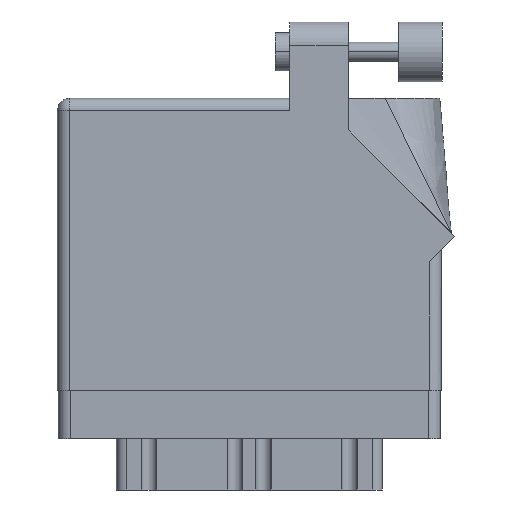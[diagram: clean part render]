
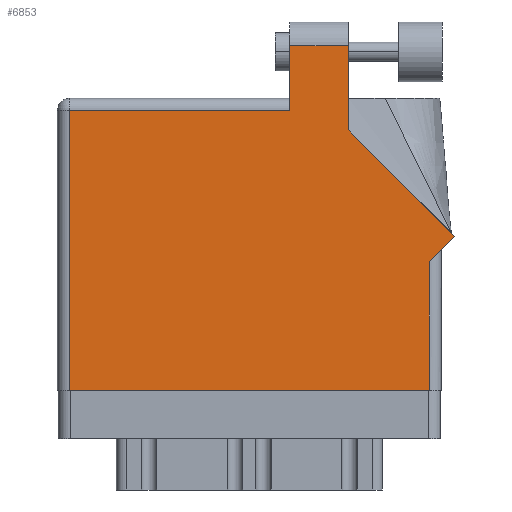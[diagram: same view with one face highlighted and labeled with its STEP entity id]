
A CAD part, front view. The second image highlights one B-rep face of the part: STEP entity #6853.
In plain terms, the highlighted face is planar.
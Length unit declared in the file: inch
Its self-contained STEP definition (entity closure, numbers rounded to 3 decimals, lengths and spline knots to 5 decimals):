
#353 = CARTESIAN_POINT ( 'NONE',  ( 1.948, 0.737, 0. ) ) ;
#829 = EDGE_CURVE ( 'NONE', #38516, #25380, #16410, .T. ) ;
#2902 = DIRECTION ( 'NONE',  ( 0., 1., 0. ) ) ;
#3990 = LINE ( 'NONE', #10843, #8149 ) ;
#4047 = DIRECTION ( 'NONE',  ( 0., -1., 0. ) ) ;
#4136 = EDGE_CURVE ( 'NONE', #24967, #4678, #3990, .T. ) ;
#4527 = VECTOR ( 'NONE', #28028, 39.37008 ) ;
#4678 = VERTEX_POINT ( 'NONE', #18419 ) ;
#5906 = EDGE_CURVE ( 'NONE', #9561, #29382, #34043, .T. ) ;
#6853 = ADVANCED_FACE ( 'NONE', ( #13841 ), #32233, .F. ) ;
#6897 = AXIS2_PLACEMENT_3D ( 'NONE', #11452, #38117, #23418 ) ;
#7195 = CARTESIAN_POINT ( 'NONE',  ( 2.01, 0.737, 0. ) ) ;
#7504 = ORIENTED_EDGE ( 'NONE', *, *, #23380, .T. ) ;
#7638 = LINE ( 'NONE', #16473, #4527 ) ;
#7779 = DIRECTION ( 'NONE',  ( 0., 1., 0. ) ) ;
#8149 = VECTOR ( 'NONE', #25350, 39.37008 ) ;
#8439 = CARTESIAN_POINT ( 'NONE',  ( 1.217, 1.805, 0. ) ) ;
#8461 = ORIENTED_EDGE ( 'NONE', *, *, #4136, .T. ) ;
#9418 = VECTOR ( 'NONE', #7779, 39.37008 ) ;
#9561 = VERTEX_POINT ( 'NONE', #8439 ) ;
#9796 = VECTOR ( 'NONE', #33236, 39.37008 ) ;
#10843 = CARTESIAN_POINT ( 'NONE',  ( 0.062, 0., 0. ) ) ;
#11318 = CARTESIAN_POINT ( 'NONE',  ( 1.948, 0.675, 0. ) ) ;
#11452 = CARTESIAN_POINT ( 'NONE',  ( 0., 1.53, 0. ) ) ;
#11966 = CARTESIAN_POINT ( 'NONE',  ( 1.217, 1.468, 0. ) ) ;
#12072 = LINE ( 'NONE', #18358, #9796 ) ;
#12632 = VECTOR ( 'NONE', #2902, 39.37008 ) ;
#13288 = DIRECTION ( 'NONE',  ( -1., 0., 0. ) ) ;
#13841 = FACE_OUTER_BOUND ( 'NONE', #28817, .T. ) ;
#15250 = ORIENTED_EDGE ( 'NONE', *, *, #22180, .T. ) ;
#15827 = CARTESIAN_POINT ( 'NONE',  ( 1.217, 1.53, 0. ) ) ;
#16410 = LINE ( 'NONE', #25608, #9418 ) ;
#16473 = CARTESIAN_POINT ( 'NONE',  ( 0., 0., 0. ) ) ;
#18358 = CARTESIAN_POINT ( 'NONE',  ( 1.217, 1.805, 0. ) ) ;
#18419 = CARTESIAN_POINT ( 'NONE',  ( 0.062, 0., 0. ) ) ;
#19212 = VERTEX_POINT ( 'NONE', #11318 ) ;
#19356 = DIRECTION ( 'NONE',  ( 0.707, 0.707, 0. ) ) ;
#19730 = LINE ( 'NONE', #35194, #34895 ) ;
#20084 = ORIENTED_EDGE ( 'NONE', *, *, #829, .T. ) ;
#21513 = CARTESIAN_POINT ( 'NONE',  ( 0., 1.468, 0. ) ) ;
#22180 = EDGE_CURVE ( 'NONE', #29382, #24967, #34233, .T. ) ;
#22627 = ORIENTED_EDGE ( 'NONE', *, *, #23321, .T. ) ;
#23281 = VECTOR ( 'NONE', #19356, 39.37008 ) ;
#23321 = EDGE_CURVE ( 'NONE', #36296, #19212, #32884, .T. ) ;
#23380 = EDGE_CURVE ( 'NONE', #19212, #27389, #30331, .T. ) ;
#23418 = DIRECTION ( 'NONE',  ( -1., 0., 0. ) ) ;
#23932 = ORIENTED_EDGE ( 'NONE', *, *, #31136, .T. ) ;
#24374 = CARTESIAN_POINT ( 'NONE',  ( 1.524, 1.36442, 0. ) ) ;
#24390 = ORIENTED_EDGE ( 'NONE', *, *, #5906, .T. ) ;
#24967 = VERTEX_POINT ( 'NONE', #28764 ) ;
#25350 = DIRECTION ( 'NONE',  ( 0., -1., 0. ) ) ;
#25380 = VERTEX_POINT ( 'NONE', #38485 ) ;
#25608 = CARTESIAN_POINT ( 'NONE',  ( 1.524, 1.36442, 0. ) ) ;
#25921 = VECTOR ( 'NONE', #4047, 39.37008 ) ;
#27389 = VERTEX_POINT ( 'NONE', #30285 ) ;
#28028 = DIRECTION ( 'NONE',  ( 1., 0., 0. ) ) ;
#28764 = CARTESIAN_POINT ( 'NONE',  ( 0.062, 1.468, 0. ) ) ;
#28817 = EDGE_LOOP ( 'NONE', ( #20084, #29443, #24390, #15250, #8461, #23932, #22627, #7504, #34879 ) ) ;
#29382 = VERTEX_POINT ( 'NONE', #11966 ) ;
#29443 = ORIENTED_EDGE ( 'NONE', *, *, #35487, .T. ) ;
#30285 = CARTESIAN_POINT ( 'NONE',  ( 2.08071, 0.80771, 0. ) ) ;
#30331 = LINE ( 'NONE', #7195, #23281 ) ;
#31136 = EDGE_CURVE ( 'NONE', #4678, #36296, #7638, .T. ) ;
#31668 = DIRECTION ( 'NONE',  ( -0.707, 0.707, 0. ) ) ;
#32233 = PLANE ( 'NONE',  #6897 ) ;
#32884 = LINE ( 'NONE', #353, #12632 ) ;
#33236 = DIRECTION ( 'NONE',  ( -1., 0., 0. ) ) ;
#34043 = LINE ( 'NONE', #15827, #25921 ) ;
#34233 = LINE ( 'NONE', #21513, #38245 ) ;
#34879 = ORIENTED_EDGE ( 'NONE', *, *, #36418, .T. ) ;
#34895 = VECTOR ( 'NONE', #31668, 39.37008 ) ;
#35194 = CARTESIAN_POINT ( 'NONE',  ( 2.08071, 0.80771, 0. ) ) ;
#35487 = EDGE_CURVE ( 'NONE', #25380, #9561, #12072, .T. ) ;
#35646 = CARTESIAN_POINT ( 'NONE',  ( 1.948, 0., 0. ) ) ;
#36296 = VERTEX_POINT ( 'NONE', #35646 ) ;
#36418 = EDGE_CURVE ( 'NONE', #27389, #38516, #19730, .T. ) ;
#38117 = DIRECTION ( 'NONE',  ( 0., 0., -1. ) ) ;
#38245 = VECTOR ( 'NONE', #13288, 39.37008 ) ;
#38485 = CARTESIAN_POINT ( 'NONE',  ( 1.524, 1.805, 0. ) ) ;
#38516 = VERTEX_POINT ( 'NONE', #24374 ) ;
